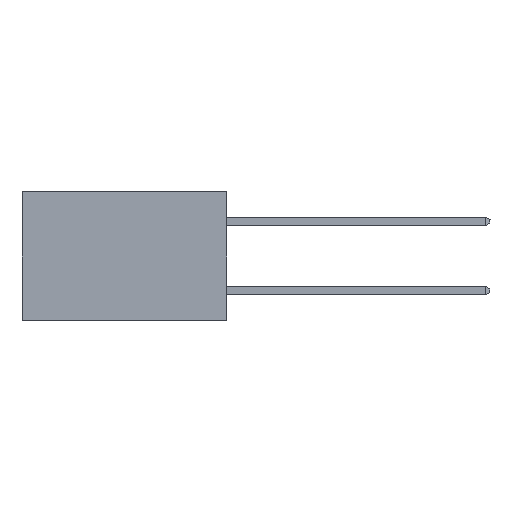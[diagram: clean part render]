
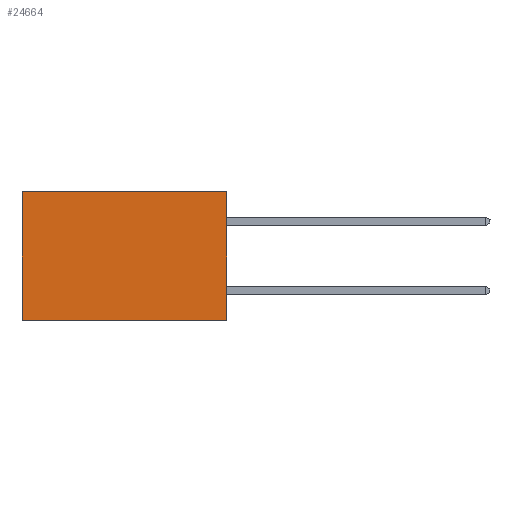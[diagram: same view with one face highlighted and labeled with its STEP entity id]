
A CAD part, left-side view. The second image highlights one B-rep face of the part: STEP entity #24664.
In plain terms, the highlighted planar face has unit normal (-1, 0, 0).
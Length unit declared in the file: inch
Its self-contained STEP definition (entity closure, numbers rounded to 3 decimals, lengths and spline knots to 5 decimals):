
#301 = CARTESIAN_POINT ( 'NONE',  ( 0.277, 0., -0.37 ) ) ;
#638 = EDGE_CURVE ( 'NONE', #12743, #33433, #20191, .T. ) ;
#3541 = CARTESIAN_POINT ( 'NONE',  ( 0.277, 0., 0. ) ) ;
#4665 = LINE ( 'NONE', #24490, #24519 ) ;
#4964 = ORIENTED_EDGE ( 'NONE', *, *, #14953, .T. ) ;
#5258 = DIRECTION ( 'NONE',  ( 0., 1., 0. ) ) ;
#5369 = AXIS2_PLACEMENT_3D ( 'NONE', #9376, #22135, #30122 ) ;
#6346 = VECTOR ( 'NONE', #20819, 39.37008 ) ;
#7828 = ORIENTED_EDGE ( 'NONE', *, *, #638, .T. ) ;
#9376 = CARTESIAN_POINT ( 'NONE',  ( 0.277, 0., -0.37 ) ) ;
#11029 = EDGE_CURVE ( 'NONE', #12743, #24402, #31981, .T. ) ;
#11990 = PLANE ( 'NONE',  #5369 ) ;
#12743 = VERTEX_POINT ( 'NONE', #13369 ) ;
#12907 = FACE_OUTER_BOUND ( 'NONE', #15738, .T. ) ;
#13369 = CARTESIAN_POINT ( 'NONE',  ( 0.277, 0., 0. ) ) ;
#13746 = VERTEX_POINT ( 'NONE', #17514 ) ;
#14953 = EDGE_CURVE ( 'NONE', #33433, #13746, #4665, .T. ) ;
#15738 = EDGE_LOOP ( 'NONE', ( #4964, #21023, #29946, #7828 ) ) ;
#17346 = LINE ( 'NONE', #20815, #31122 ) ;
#17376 = VECTOR ( 'NONE', #25011, 39.37008 ) ;
#17514 = CARTESIAN_POINT ( 'NONE',  ( 0.277, 0.59, -0.37 ) ) ;
#17595 = CARTESIAN_POINT ( 'NONE',  ( 0.277, 0.59, 0. ) ) ;
#20191 = LINE ( 'NONE', #3541, #6346 ) ;
#20298 = EDGE_CURVE ( 'NONE', #24402, #13746, #17346, .T. ) ;
#20815 = CARTESIAN_POINT ( 'NONE',  ( 0.277, 0., -0.37 ) ) ;
#20819 = DIRECTION ( 'NONE',  ( 0., 1., 0. ) ) ;
#21023 = ORIENTED_EDGE ( 'NONE', *, *, #20298, .F. ) ;
#22017 = DIRECTION ( 'NONE',  ( 0., 0., -1. ) ) ;
#22135 = DIRECTION ( 'NONE',  ( 1., 0., 0. ) ) ;
#22409 = CARTESIAN_POINT ( 'NONE',  ( 0.277, 0., -0.37 ) ) ;
#24402 = VERTEX_POINT ( 'NONE', #301 ) ;
#24490 = CARTESIAN_POINT ( 'NONE',  ( 0.277, 0.59, -0.37 ) ) ;
#24519 = VECTOR ( 'NONE', #22017, 39.37008 ) ;
#24664 = ADVANCED_FACE ( 'NONE', ( #12907 ), #11990, .F. ) ;
#25011 = DIRECTION ( 'NONE',  ( 0., 0., -1. ) ) ;
#29946 = ORIENTED_EDGE ( 'NONE', *, *, #11029, .F. ) ;
#30122 = DIRECTION ( 'NONE',  ( 0., 0., -1. ) ) ;
#31122 = VECTOR ( 'NONE', #5258, 39.37008 ) ;
#31981 = LINE ( 'NONE', #22409, #17376 ) ;
#33433 = VERTEX_POINT ( 'NONE', #17595 ) ;
